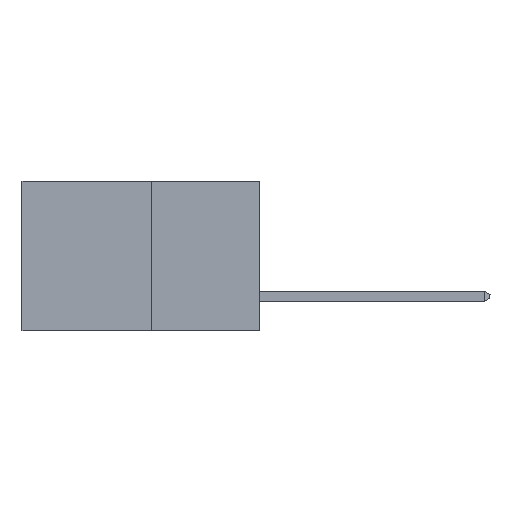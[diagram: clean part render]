
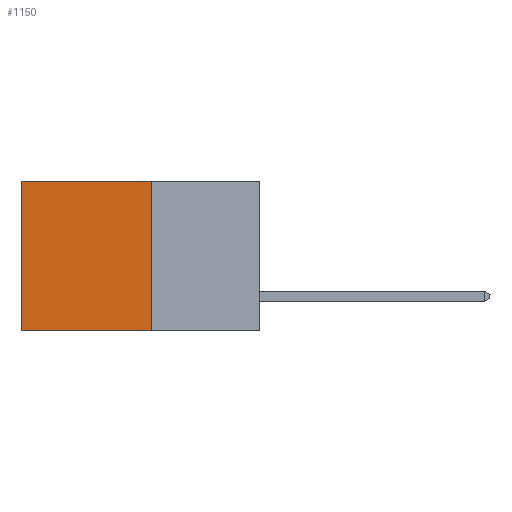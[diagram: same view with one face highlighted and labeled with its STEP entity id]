
A CAD part, left-side view. The second image highlights one B-rep face of the part: STEP entity #1150.
In plain terms, the highlighted planar face has unit normal (-1, 0, 0).
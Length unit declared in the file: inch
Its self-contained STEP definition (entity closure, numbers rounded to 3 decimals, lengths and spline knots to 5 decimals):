
#664 = CARTESIAN_POINT ( 'NONE',  ( 0.277, 0.27, -0.37 ) ) ;
#921 = ORIENTED_EDGE ( 'NONE', *, *, #11449, .T. ) ;
#958 = FACE_OUTER_BOUND ( 'NONE', #3704, .T. ) ;
#1150 = ADVANCED_FACE ( 'NONE', ( #958 ), #5648, .F. ) ;
#1254 = AXIS2_PLACEMENT_3D ( 'NONE', #4847, #4817, #4780 ) ;
#1664 = ORIENTED_EDGE ( 'NONE', *, *, #4454, .F. ) ;
#1880 = LINE ( 'NONE', #3301, #13906 ) ;
#2157 = VERTEX_POINT ( 'NONE', #13178 ) ;
#2883 = VERTEX_POINT ( 'NONE', #3439 ) ;
#3264 = CARTESIAN_POINT ( 'NONE',  ( 0.277, 0.59, -0.37 ) ) ;
#3301 = CARTESIAN_POINT ( 'NONE',  ( 0.277, 0.27, -0.37 ) ) ;
#3439 = CARTESIAN_POINT ( 'NONE',  ( 0.277, 0.59, 0. ) ) ;
#3704 = EDGE_LOOP ( 'NONE', ( #921, #13697, #1664, #11012 ) ) ;
#4086 = VECTOR ( 'NONE', #8415, 39.37008 ) ;
#4221 = CARTESIAN_POINT ( 'NONE',  ( 0.277, 0.27, 0. ) ) ;
#4454 = EDGE_CURVE ( 'NONE', #2157, #5979, #4820, .T. ) ;
#4780 = DIRECTION ( 'NONE',  ( 0., 0., -1. ) ) ;
#4817 = DIRECTION ( 'NONE',  ( 1., 0., 0. ) ) ;
#4820 = LINE ( 'NONE', #8564, #14064 ) ;
#4847 = CARTESIAN_POINT ( 'NONE',  ( 0.277, 0.27, -0.37 ) ) ;
#4966 = CARTESIAN_POINT ( 'NONE',  ( 0.277, 0.59, -0.37 ) ) ;
#5079 = DIRECTION ( 'NONE',  ( 0., 0., -1. ) ) ;
#5648 = PLANE ( 'NONE',  #1254 ) ;
#5673 = DIRECTION ( 'NONE',  ( 0., 1., 0. ) ) ;
#5979 = VERTEX_POINT ( 'NONE', #664 ) ;
#7193 = LINE ( 'NONE', #4966, #4086 ) ;
#7377 = LINE ( 'NONE', #4221, #10100 ) ;
#8415 = DIRECTION ( 'NONE',  ( 0., 0., -1. ) ) ;
#8564 = CARTESIAN_POINT ( 'NONE',  ( 0.277, 0.27, -0.37 ) ) ;
#10034 = EDGE_CURVE ( 'NONE', #5979, #11826, #1880, .T. ) ;
#10100 = VECTOR ( 'NONE', #13524, 39.37008 ) ;
#10534 = EDGE_CURVE ( 'NONE', #2157, #2883, #7377, .T. ) ;
#11012 = ORIENTED_EDGE ( 'NONE', *, *, #10534, .T. ) ;
#11449 = EDGE_CURVE ( 'NONE', #2883, #11826, #7193, .T. ) ;
#11826 = VERTEX_POINT ( 'NONE', #3264 ) ;
#13178 = CARTESIAN_POINT ( 'NONE',  ( 0.277, 0.27, 0. ) ) ;
#13524 = DIRECTION ( 'NONE',  ( 0., 1., 0. ) ) ;
#13697 = ORIENTED_EDGE ( 'NONE', *, *, #10034, .F. ) ;
#13906 = VECTOR ( 'NONE', #5673, 39.37008 ) ;
#14064 = VECTOR ( 'NONE', #5079, 39.37008 ) ;
